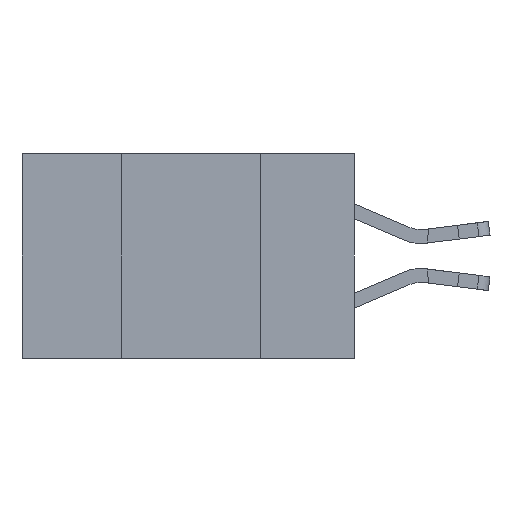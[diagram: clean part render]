
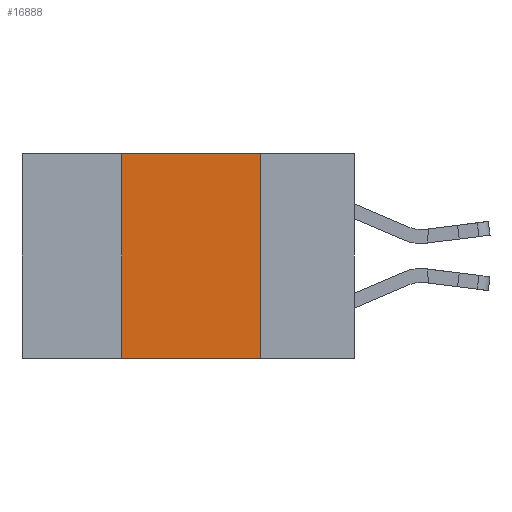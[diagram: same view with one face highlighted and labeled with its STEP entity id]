
A CAD part, left-side view. The second image highlights one B-rep face of the part: STEP entity #16888.
In plain terms, the highlighted planar face has unit normal (-1, 0, 0).
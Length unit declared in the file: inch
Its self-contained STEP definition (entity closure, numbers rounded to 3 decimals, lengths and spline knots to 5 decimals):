
#601 = CARTESIAN_POINT ( 'NONE',  ( 0., 0.17, -0.37 ) ) ;
#1104 = EDGE_CURVE ( 'NONE', #15893, #1868, #11872, .T. ) ;
#1255 = CARTESIAN_POINT ( 'NONE',  ( 0., 0.42, 0. ) ) ;
#1560 = ORIENTED_EDGE ( 'NONE', *, *, #9095, .F. ) ;
#1868 = VERTEX_POINT ( 'NONE', #1255 ) ;
#2443 = LINE ( 'NONE', #10605, #11984 ) ;
#2605 = DIRECTION ( 'NONE',  ( 0., 0., -1. ) ) ;
#2613 = AXIS2_PLACEMENT_3D ( 'NONE', #12509, #15140, #15042 ) ;
#4240 = CARTESIAN_POINT ( 'NONE',  ( 0., 0.42, -0.37 ) ) ;
#4689 = FACE_OUTER_BOUND ( 'NONE', #16968, .T. ) ;
#5257 = DIRECTION ( 'NONE',  ( 0., -1., 0. ) ) ;
#5513 = EDGE_CURVE ( 'NONE', #15893, #13893, #16337, .T. ) ;
#7571 = VECTOR ( 'NONE', #9340, 39.37008 ) ;
#7773 = LINE ( 'NONE', #11858, #8952 ) ;
#8543 = VECTOR ( 'NONE', #14662, 39.37008 ) ;
#8641 = ORIENTED_EDGE ( 'NONE', *, *, #14388, .F. ) ;
#8952 = VECTOR ( 'NONE', #5257, 39.37008 ) ;
#9095 = EDGE_CURVE ( 'NONE', #12156, #13893, #2443, .T. ) ;
#9340 = DIRECTION ( 'NONE',  ( 0., -1., 0. ) ) ;
#9829 = PLANE ( 'NONE',  #2613 ) ;
#10605 = CARTESIAN_POINT ( 'NONE',  ( 0., 0.17, -0.37 ) ) ;
#11497 = ORIENTED_EDGE ( 'NONE', *, *, #1104, .F. ) ;
#11530 = CARTESIAN_POINT ( 'NONE',  ( 0., 0.42, -0.37 ) ) ;
#11858 = CARTESIAN_POINT ( 'NONE',  ( 0., 0.6, 0. ) ) ;
#11872 = LINE ( 'NONE', #4240, #8543 ) ;
#11984 = VECTOR ( 'NONE', #2605, 39.37008 ) ;
#12156 = VERTEX_POINT ( 'NONE', #14337 ) ;
#12509 = CARTESIAN_POINT ( 'NONE',  ( 0., 0.6, 0. ) ) ;
#13893 = VERTEX_POINT ( 'NONE', #601 ) ;
#14337 = CARTESIAN_POINT ( 'NONE',  ( 0., 0.17, 0. ) ) ;
#14388 = EDGE_CURVE ( 'NONE', #1868, #12156, #7773, .T. ) ;
#14662 = DIRECTION ( 'NONE',  ( 0., 0., 1. ) ) ;
#15042 = DIRECTION ( 'NONE',  ( 0., 0., -1. ) ) ;
#15140 = DIRECTION ( 'NONE',  ( 1., 0., 0. ) ) ;
#15893 = VERTEX_POINT ( 'NONE', #11530 ) ;
#15967 = CARTESIAN_POINT ( 'NONE',  ( 0., 0.6, -0.37 ) ) ;
#16337 = LINE ( 'NONE', #15967, #7571 ) ;
#16395 = ORIENTED_EDGE ( 'NONE', *, *, #5513, .T. ) ;
#16888 = ADVANCED_FACE ( 'NONE', ( #4689 ), #9829, .F. ) ;
#16968 = EDGE_LOOP ( 'NONE', ( #1560, #8641, #11497, #16395 ) ) ;
